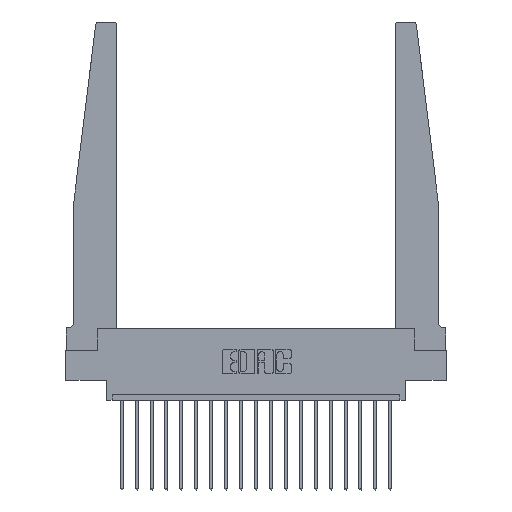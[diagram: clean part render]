
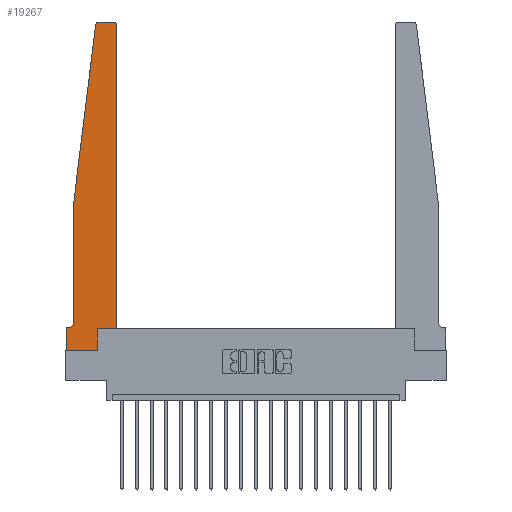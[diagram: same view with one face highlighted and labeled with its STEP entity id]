
A CAD part, top view. The second image highlights one B-rep face of the part: STEP entity #19267.
In plain terms, the highlighted planar face has unit normal (0, 0, 1).
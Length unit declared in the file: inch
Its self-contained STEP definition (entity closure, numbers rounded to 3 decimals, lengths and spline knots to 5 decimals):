
#160 = DIRECTION ( 'NONE',  ( -1., 0., 0. ) ) ;
#239 = DIRECTION ( 'NONE',  ( 0., 1., 0. ) ) ;
#303 = CARTESIAN_POINT ( 'NONE',  ( 0.27653, 2.75, 0.37 ) ) ;
#439 = DIRECTION ( 'NONE',  ( 1., 0., 0. ) ) ;
#781 = EDGE_CURVE ( 'NONE', #14221, #3537, #3687, .T. ) ;
#1044 = VERTEX_POINT ( 'NONE', #1520 ) ;
#1520 = CARTESIAN_POINT ( 'NONE',  ( 0.2605, 0.18, 0.37 ) ) ;
#1547 = EDGE_CURVE ( 'NONE', #14112, #2509, #13285, .T. ) ;
#1735 = ORIENTED_EDGE ( 'NONE', *, *, #2765, .T. ) ;
#1992 = VECTOR ( 'NONE', #11559, 39.37008 ) ;
#2509 = VERTEX_POINT ( 'NONE', #17348 ) ;
#2536 = VERTEX_POINT ( 'NONE', #5074 ) ;
#2732 = VECTOR ( 'NONE', #15950, 39.37008 ) ;
#2765 = EDGE_CURVE ( 'NONE', #2509, #5219, #8941, .T. ) ;
#2767 = VECTOR ( 'NONE', #239, 39.37008 ) ;
#3063 = PLANE ( 'NONE',  #15858 ) ;
#3146 = CARTESIAN_POINT ( 'NONE',  ( 0.015, 0.2375, 0.37 ) ) ;
#3339 = EDGE_CURVE ( 'NONE', #4974, #14221, #14926, .T. ) ;
#3508 = DIRECTION ( 'NONE',  ( 1., 0., 0. ) ) ;
#3537 = VERTEX_POINT ( 'NONE', #13496 ) ;
#3687 = LINE ( 'NONE', #8491, #2732 ) ;
#4052 = CARTESIAN_POINT ( 'NONE',  ( 0.425, 0.18, 0.37 ) ) ;
#4203 = CARTESIAN_POINT ( 'NONE',  ( 0.065, 0.2375, 0.37 ) ) ;
#4285 = ORIENTED_EDGE ( 'NONE', *, *, #16047, .T. ) ;
#4785 = DIRECTION ( 'NONE',  ( -1., 0., 0. ) ) ;
#4844 = CARTESIAN_POINT ( 'NONE',  ( 0.27653, 2.72, 0.37 ) ) ;
#4974 = VERTEX_POINT ( 'NONE', #5603 ) ;
#5011 = DIRECTION ( 'NONE',  ( 1., 0., 0. ) ) ;
#5023 = CIRCLE ( 'NONE', #19079, 0.03 ) ;
#5074 = CARTESIAN_POINT ( 'NONE',  ( 0.425, 2.72, 0.37 ) ) ;
#5219 = VERTEX_POINT ( 'NONE', #13571 ) ;
#5412 = DIRECTION ( 'NONE',  ( 0., 1., 0. ) ) ;
#5603 = CARTESIAN_POINT ( 'NONE',  ( 0.015, 0.1875, 0.37 ) ) ;
#5786 = AXIS2_PLACEMENT_3D ( 'NONE', #4844, #9740, #15965 ) ;
#6150 = LINE ( 'NONE', #12373, #10440 ) ;
#6465 = EDGE_LOOP ( 'NONE', ( #4285, #7665, #1735, #19141, #17808, #16345, #19207, #12745, #14160, #16816, #9889, #19090 ) ) ;
#6492 = CARTESIAN_POINT ( 'NONE',  ( 0.2605, 0.18, 0.37 ) ) ;
#6831 = VERTEX_POINT ( 'NONE', #10035 ) ;
#7328 = VECTOR ( 'NONE', #20086, 39.37008 ) ;
#7362 = CARTESIAN_POINT ( 'NONE',  ( 0., 0.1875, 0.37 ) ) ;
#7370 = CARTESIAN_POINT ( 'NONE',  ( 0.065, 1.25, 0.37 ) ) ;
#7436 = CARTESIAN_POINT ( 'NONE',  ( 0.2605, 0., 0.37 ) ) ;
#7594 = CARTESIAN_POINT ( 'NONE',  ( 0.425, 0.18, 0.37 ) ) ;
#7665 = ORIENTED_EDGE ( 'NONE', *, *, #1547, .T. ) ;
#8187 = VECTOR ( 'NONE', #18451, 39.37008 ) ;
#8491 = CARTESIAN_POINT ( 'NONE',  ( 0., 0., 0.37 ) ) ;
#8500 = EDGE_CURVE ( 'NONE', #9141, #2536, #6150, .T. ) ;
#8941 = LINE ( 'NONE', #10571, #8187 ) ;
#9141 = VERTEX_POINT ( 'NONE', #4052 ) ;
#9315 = DIRECTION ( 'NONE',  ( 0., 0., 1. ) ) ;
#9740 = DIRECTION ( 'NONE',  ( 0., 0., 1. ) ) ;
#9751 = LINE ( 'NONE', #6492, #2767 ) ;
#9889 = ORIENTED_EDGE ( 'NONE', *, *, #8500, .T. ) ;
#10035 = CARTESIAN_POINT ( 'NONE',  ( 0.395, 2.75, 0.37 ) ) ;
#10070 = EDGE_CURVE ( 'NONE', #5219, #19166, #15126, .T. ) ;
#10440 = VECTOR ( 'NONE', #5412, 39.37008 ) ;
#10571 = CARTESIAN_POINT ( 'NONE',  ( 0.065, 1.25, 0.37 ) ) ;
#10862 = VECTOR ( 'NONE', #3508, 39.37008 ) ;
#11559 = DIRECTION ( 'NONE',  ( -1., 0., 0. ) ) ;
#12373 = CARTESIAN_POINT ( 'NONE',  ( 0.425, 0.18, 0.37 ) ) ;
#12615 = CARTESIAN_POINT ( 'NONE',  ( 0.395, 2.72, 0.37 ) ) ;
#12622 = CIRCLE ( 'NONE', #15869, 0.05 ) ;
#12745 = ORIENTED_EDGE ( 'NONE', *, *, #13793, .T. ) ;
#13285 = CIRCLE ( 'NONE', #5786, 0.03 ) ;
#13496 = CARTESIAN_POINT ( 'NONE',  ( 0., 0., 0.37 ) ) ;
#13571 = CARTESIAN_POINT ( 'NONE',  ( 0.065, 1.25, 0.37 ) ) ;
#13601 = DIRECTION ( 'NONE',  ( 0., -1., 0. ) ) ;
#13793 = EDGE_CURVE ( 'NONE', #3537, #15970, #17241, .T. ) ;
#14084 = DIRECTION ( 'NONE',  ( 0., 0., -1. ) ) ;
#14112 = VERTEX_POINT ( 'NONE', #303 ) ;
#14160 = ORIENTED_EDGE ( 'NONE', *, *, #16502, .T. ) ;
#14221 = VERTEX_POINT ( 'NONE', #7362 ) ;
#14926 = LINE ( 'NONE', #17910, #1992 ) ;
#15126 = LINE ( 'NONE', #7370, #19948 ) ;
#15152 = LINE ( 'NONE', #7594, #7328 ) ;
#15291 = LINE ( 'NONE', #17045, #19094 ) ;
#15491 = EDGE_CURVE ( 'NONE', #2536, #6831, #5023, .T. ) ;
#15539 = FACE_OUTER_BOUND ( 'NONE', #6465, .T. ) ;
#15637 = CARTESIAN_POINT ( 'NONE',  ( 0., 0.1875, 0.37 ) ) ;
#15858 = AXIS2_PLACEMENT_3D ( 'NONE', #15637, #9315, #5011 ) ;
#15869 = AXIS2_PLACEMENT_3D ( 'NONE', #3146, #14084, #4785 ) ;
#15950 = DIRECTION ( 'NONE',  ( 0., -1., 0. ) ) ;
#15965 = DIRECTION ( 'NONE',  ( 1., 0., 0. ) ) ;
#15970 = VERTEX_POINT ( 'NONE', #7436 ) ;
#16047 = EDGE_CURVE ( 'NONE', #6831, #14112, #15291, .T. ) ;
#16345 = ORIENTED_EDGE ( 'NONE', *, *, #3339, .T. ) ;
#16502 = EDGE_CURVE ( 'NONE', #15970, #1044, #9751, .T. ) ;
#16816 = ORIENTED_EDGE ( 'NONE', *, *, #17344, .T. ) ;
#17045 = CARTESIAN_POINT ( 'NONE',  ( 0.25, 2.75, 0.37 ) ) ;
#17241 = LINE ( 'NONE', #19260, #10862 ) ;
#17344 = EDGE_CURVE ( 'NONE', #1044, #9141, #15152, .T. ) ;
#17348 = CARTESIAN_POINT ( 'NONE',  ( 0.24675, 2.72367, 0.37 ) ) ;
#17808 = ORIENTED_EDGE ( 'NONE', *, *, #19826, .T. ) ;
#17910 = CARTESIAN_POINT ( 'NONE',  ( 0.065, 0.1875, 0.37 ) ) ;
#18451 = DIRECTION ( 'NONE',  ( -0.122, -0.992, 0. ) ) ;
#19068 = DIRECTION ( 'NONE',  ( 0., 0., 1. ) ) ;
#19079 = AXIS2_PLACEMENT_3D ( 'NONE', #12615, #19068, #439 ) ;
#19090 = ORIENTED_EDGE ( 'NONE', *, *, #15491, .T. ) ;
#19094 = VECTOR ( 'NONE', #160, 39.37008 ) ;
#19141 = ORIENTED_EDGE ( 'NONE', *, *, #10070, .T. ) ;
#19166 = VERTEX_POINT ( 'NONE', #4203 ) ;
#19207 = ORIENTED_EDGE ( 'NONE', *, *, #781, .T. ) ;
#19260 = CARTESIAN_POINT ( 'NONE',  ( 0., 0., 0.37 ) ) ;
#19267 = ADVANCED_FACE ( 'NONE', ( #15539 ), #3063, .T. ) ;
#19826 = EDGE_CURVE ( 'NONE', #19166, #4974, #12622, .T. ) ;
#19948 = VECTOR ( 'NONE', #13601, 39.37008 ) ;
#20086 = DIRECTION ( 'NONE',  ( 1., 0., 0. ) ) ;
